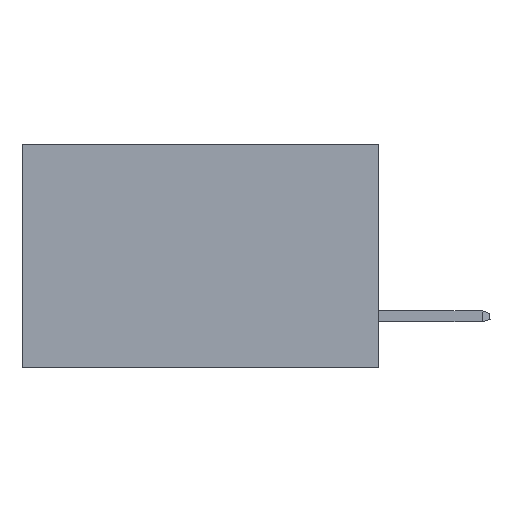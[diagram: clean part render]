
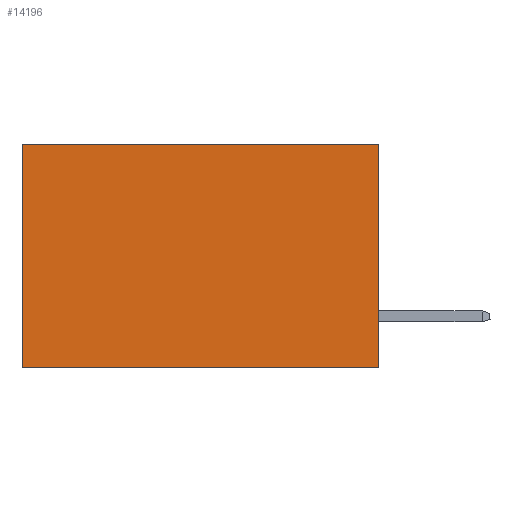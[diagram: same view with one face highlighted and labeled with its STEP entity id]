
A CAD part, left-side view. The second image highlights one B-rep face of the part: STEP entity #14196.
In plain terms, the highlighted planar face has unit normal (-1, 0, 0).
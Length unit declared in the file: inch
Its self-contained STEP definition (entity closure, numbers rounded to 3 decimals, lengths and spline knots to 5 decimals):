
#575 = VERTEX_POINT ( 'NONE', #9937 ) ;
#2328 = VECTOR ( 'NONE', #17118, 39.37008 ) ;
#2483 = DIRECTION ( 'NONE',  ( 0., 0., -1. ) ) ;
#2938 = EDGE_LOOP ( 'NONE', ( #19761, #22765, #11727, #10729 ) ) ;
#5699 = DIRECTION ( 'NONE',  ( 0., 0., -1. ) ) ;
#5976 = CARTESIAN_POINT ( 'NONE',  ( 0.277, 0.59, 0. ) ) ;
#6036 = EDGE_CURVE ( 'NONE', #9515, #15613, #26456, .T. ) ;
#7956 = PLANE ( 'NONE',  #24286 ) ;
#8070 = LINE ( 'NONE', #10590, #19778 ) ;
#8562 = VECTOR ( 'NONE', #2483, 39.37008 ) ;
#9515 = VERTEX_POINT ( 'NONE', #24842 ) ;
#9937 = CARTESIAN_POINT ( 'NONE',  ( 0.277, 0., 0. ) ) ;
#10545 = FACE_OUTER_BOUND ( 'NONE', #2938, .T. ) ;
#10590 = CARTESIAN_POINT ( 'NONE',  ( 0.277, 0., 0. ) ) ;
#10729 = ORIENTED_EDGE ( 'NONE', *, *, #25016, .T. ) ;
#10778 = LINE ( 'NONE', #18927, #8562 ) ;
#11145 = VERTEX_POINT ( 'NONE', #5976 ) ;
#11727 = ORIENTED_EDGE ( 'NONE', *, *, #27767, .F. ) ;
#12026 = CARTESIAN_POINT ( 'NONE',  ( 0.277, 0., -0.37 ) ) ;
#12936 = DIRECTION ( 'NONE',  ( 0., 1., 0. ) ) ;
#14196 = ADVANCED_FACE ( 'NONE', ( #10545 ), #7956, .F. ) ;
#14297 = DIRECTION ( 'NONE',  ( 0., 0., -1. ) ) ;
#15043 = CARTESIAN_POINT ( 'NONE',  ( 0.277, 0., -0.37 ) ) ;
#15613 = VERTEX_POINT ( 'NONE', #22394 ) ;
#17118 = DIRECTION ( 'NONE',  ( 0., 1., 0. ) ) ;
#17268 = CARTESIAN_POINT ( 'NONE',  ( 0.277, 0., -0.37 ) ) ;
#18927 = CARTESIAN_POINT ( 'NONE',  ( 0.277, 0.59, -0.37 ) ) ;
#19726 = DIRECTION ( 'NONE',  ( 1., 0., 0. ) ) ;
#19761 = ORIENTED_EDGE ( 'NONE', *, *, #29676, .T. ) ;
#19778 = VECTOR ( 'NONE', #12936, 39.37008 ) ;
#21079 = LINE ( 'NONE', #12026, #22534 ) ;
#22394 = CARTESIAN_POINT ( 'NONE',  ( 0.277, 0.59, -0.37 ) ) ;
#22534 = VECTOR ( 'NONE', #14297, 39.37008 ) ;
#22765 = ORIENTED_EDGE ( 'NONE', *, *, #6036, .F. ) ;
#24286 = AXIS2_PLACEMENT_3D ( 'NONE', #15043, #19726, #5699 ) ;
#24842 = CARTESIAN_POINT ( 'NONE',  ( 0.277, 0., -0.37 ) ) ;
#25016 = EDGE_CURVE ( 'NONE', #575, #11145, #8070, .T. ) ;
#26456 = LINE ( 'NONE', #17268, #2328 ) ;
#27767 = EDGE_CURVE ( 'NONE', #575, #9515, #21079, .T. ) ;
#29676 = EDGE_CURVE ( 'NONE', #11145, #15613, #10778, .T. ) ;
